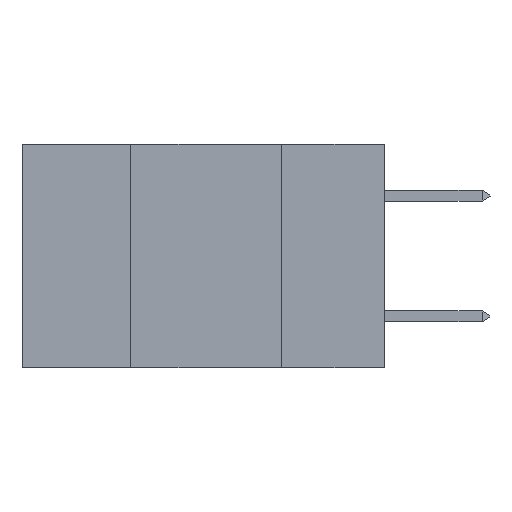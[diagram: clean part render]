
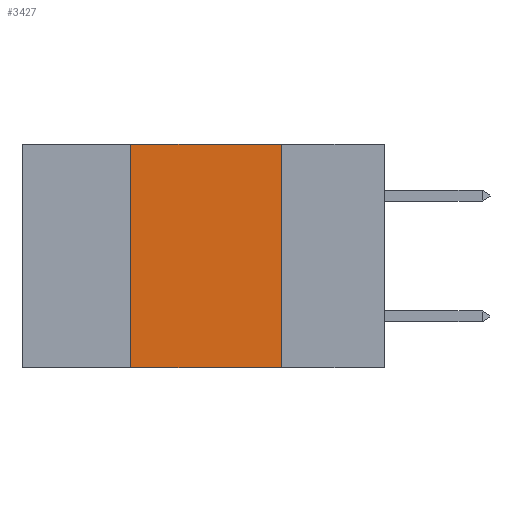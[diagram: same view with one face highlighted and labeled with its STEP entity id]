
A CAD part, left-side view. The second image highlights one B-rep face of the part: STEP entity #3427.
In plain terms, the highlighted planar face has unit normal (-1, 0, 0).
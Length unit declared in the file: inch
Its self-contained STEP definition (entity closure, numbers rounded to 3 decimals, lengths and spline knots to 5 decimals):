
#110 = LINE ( 'NONE', #18117, #17172 ) ;
#2078 = LINE ( 'NONE', #8420, #16952 ) ;
#2275 = VERTEX_POINT ( 'NONE', #14400 ) ;
#3427 = ADVANCED_FACE ( 'NONE', ( #6667 ), #18623, .F. ) ;
#3441 = CARTESIAN_POINT ( 'NONE',  ( 0., 0.42, -0.37 ) ) ;
#4100 = CARTESIAN_POINT ( 'NONE',  ( 0., 0.17, 0. ) ) ;
#5008 = LINE ( 'NONE', #4100, #13673 ) ;
#5201 = CARTESIAN_POINT ( 'NONE',  ( 0., 0.6, 0. ) ) ;
#5246 = EDGE_CURVE ( 'NONE', #5363, #9487, #5008, .T. ) ;
#5363 = VERTEX_POINT ( 'NONE', #7433 ) ;
#5788 = EDGE_CURVE ( 'NONE', #2275, #5363, #9066, .T. ) ;
#6667 = FACE_OUTER_BOUND ( 'NONE', #13909, .T. ) ;
#7158 = ORIENTED_EDGE ( 'NONE', *, *, #8115, .T. ) ;
#7433 = CARTESIAN_POINT ( 'NONE',  ( 0., 0.17, 0. ) ) ;
#7546 = DIRECTION ( 'NONE',  ( 0., -1., 0. ) ) ;
#7602 = DIRECTION ( 'NONE',  ( 0., -1., 0. ) ) ;
#8041 = VECTOR ( 'NONE', #7602, 39.37008 ) ;
#8115 = EDGE_CURVE ( 'NONE', #10706, #9487, #110, .T. ) ;
#8270 = AXIS2_PLACEMENT_3D ( 'NONE', #5201, #11198, #17153 ) ;
#8420 = CARTESIAN_POINT ( 'NONE',  ( 0., 0.42, 0. ) ) ;
#8508 = DIRECTION ( 'NONE',  ( 0., 0., -1. ) ) ;
#9066 = LINE ( 'NONE', #12021, #8041 ) ;
#9487 = VERTEX_POINT ( 'NONE', #10496 ) ;
#9603 = DIRECTION ( 'NONE',  ( 0., 0., 1. ) ) ;
#10496 = CARTESIAN_POINT ( 'NONE',  ( 0., 0.17, -0.37 ) ) ;
#10706 = VERTEX_POINT ( 'NONE', #3441 ) ;
#11198 = DIRECTION ( 'NONE',  ( 1., 0., 0. ) ) ;
#12021 = CARTESIAN_POINT ( 'NONE',  ( 0., 0.6, 0. ) ) ;
#13173 = EDGE_CURVE ( 'NONE', #10706, #2275, #2078, .T. ) ;
#13334 = ORIENTED_EDGE ( 'NONE', *, *, #5788, .F. ) ;
#13673 = VECTOR ( 'NONE', #8508, 39.37008 ) ;
#13909 = EDGE_LOOP ( 'NONE', ( #14930, #13334, #17324, #7158 ) ) ;
#14400 = CARTESIAN_POINT ( 'NONE',  ( 0., 0.42, 0. ) ) ;
#14930 = ORIENTED_EDGE ( 'NONE', *, *, #5246, .F. ) ;
#16952 = VECTOR ( 'NONE', #9603, 39.37008 ) ;
#17153 = DIRECTION ( 'NONE',  ( 0., 0., -1. ) ) ;
#17172 = VECTOR ( 'NONE', #7546, 39.37008 ) ;
#17324 = ORIENTED_EDGE ( 'NONE', *, *, #13173, .F. ) ;
#18117 = CARTESIAN_POINT ( 'NONE',  ( 0., 0.6, -0.37 ) ) ;
#18623 = PLANE ( 'NONE',  #8270 ) ;
